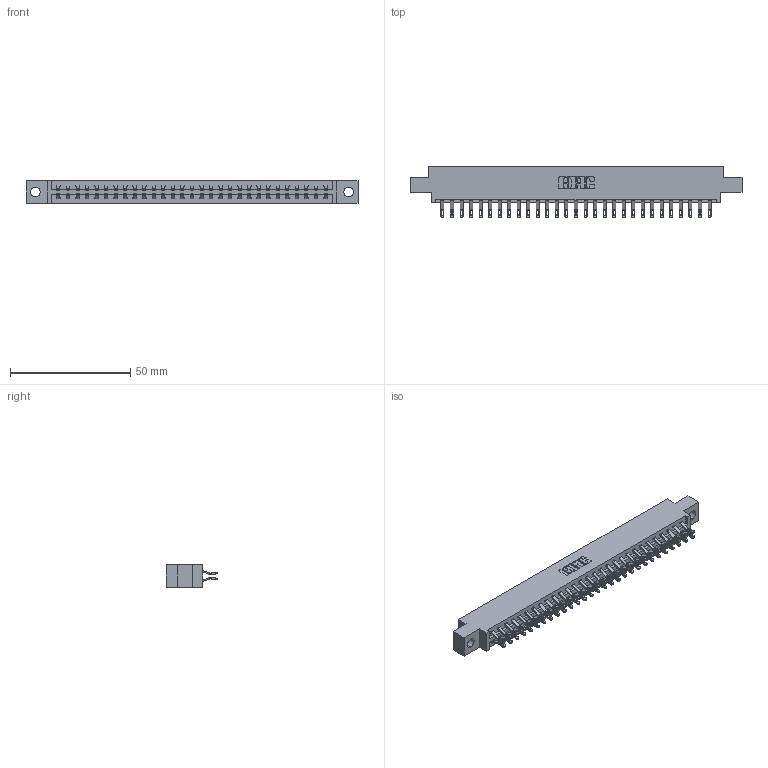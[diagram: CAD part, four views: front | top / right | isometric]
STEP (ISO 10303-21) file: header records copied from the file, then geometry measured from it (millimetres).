
FILE_DESCRIPTION (( 'STEP AP203' ), '1' );
FILE_NAME ('337-058-555-804.STEP', '2018-08-10T05:59:40', ( '' ), ( '' ), 'SwSTEP 2.0', 'SolidWorks 2016', '' );
FILE_SCHEMA (( 'CONFIG_CONTROL_DESIGN' ));
Length unit declared in the file: inch
Products named in the file (3): 345-292-001_555 Tail; 337-058-555-804; 337 Part_0.170 Offset - 0.156 Dia-TH
Assembly tree (59 placements, depth 2):
  337-058-555-804
    337 Part_0.170 Offset - 0.156 Dia-TH
    345-292-001_555 Tail  x58
Bounding box: 137.92 x 21.47 x 9.4 mm (x, y, z)
Volume: 14325.1 mm3; surface area: 16607.5 mm2
Topology: 59 solids, 59 shells, 3598 faces, 11285 edges, 7522 vertices
Faces by surface type: plane 2162, cylinder 1436
Entity records: 24627 total; most frequent: CARTESIAN_POINT 4196, ORIENTED_EDGE 4102, DIRECTION 3563, EDGE_CURVE 2051, LINE 1903, VECTOR 1903, VERTEX_POINT 1366, AXIS2_PLACEMENT_3D 830
